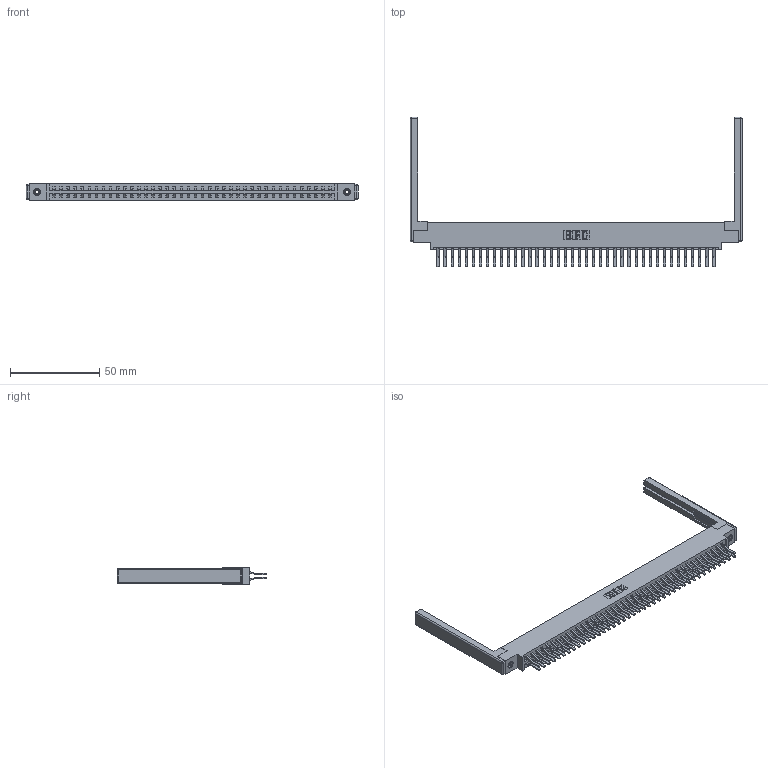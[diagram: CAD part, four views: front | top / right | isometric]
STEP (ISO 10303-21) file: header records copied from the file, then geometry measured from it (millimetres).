
FILE_DESCRIPTION (( 'STEP AP203' ), '1' );
FILE_NAME ('387-080-560-868.STEP', '2019-10-22T23:04:06', ( '' ), ( '' ), 'SwSTEP 2.0', 'SolidWorks 2016', '' );
FILE_SCHEMA (( 'CONFIG_CONTROL_DESIGN' ));
Length unit declared in the file: inch
Products named in the file (5): 337 Part_0.170 Offset - 0.156 Dia-TI; 307-220-068; 387-080-560-868; 345-250-001_345-250-001-102; 345-292-001_560 Tail
Assembly tree (85 placements, depth 2):
  387-080-560-868
    337 Part_0.170 Offset - 0.156 Dia-TI
    345-292-001_560 Tail  x80
    345-250-001_345-250-001-102  x2
    307-220-068  x2
Bounding box: 185.93 x 83.84 x 9.4 mm (x, y, z)
Volume: 24359.6 mm3; surface area: 28222 mm2
Topology: 85 solids, 85 shells, 4752 faces, 14073 edges, 9254 vertices
Faces by surface type: plane 3202, cylinder 1526, cone 12, sphere 8, torus 4
Entity records: 34252 total; most frequent: CARTESIAN_POINT 5739, ORIENTED_EDGE 5664, DIRECTION 4958, EDGE_CURVE 2832, LINE 2650, VECTOR 2650, VERTEX_POINT 1878, AXIS2_PLACEMENT_3D 1154
